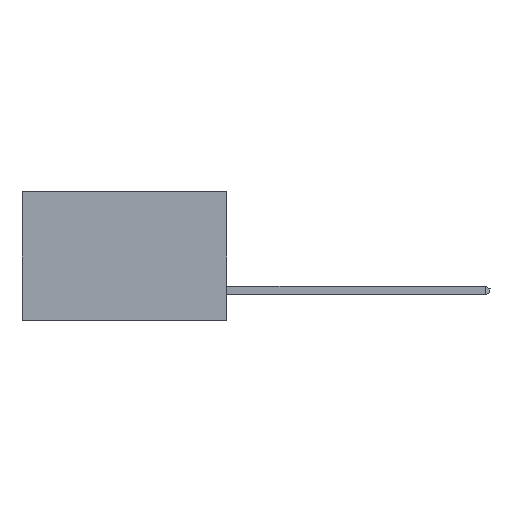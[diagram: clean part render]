
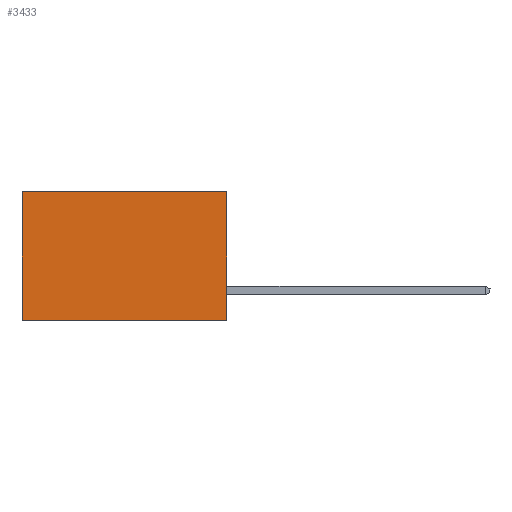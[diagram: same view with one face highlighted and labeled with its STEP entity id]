
A CAD part, left-side view. The second image highlights one B-rep face of the part: STEP entity #3433.
In plain terms, the highlighted planar face has unit normal (-1, 0, 0).
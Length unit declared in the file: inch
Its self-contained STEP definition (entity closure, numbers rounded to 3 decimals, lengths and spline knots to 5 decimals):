
#460 = ORIENTED_EDGE ( 'NONE', *, *, #3044, .F. ) ;
#635 = EDGE_CURVE ( 'NONE', #4662, #4402, #11869, .T. ) ;
#677 = ORIENTED_EDGE ( 'NONE', *, *, #10518, .T. ) ;
#2318 = AXIS2_PLACEMENT_3D ( 'NONE', #15394, #14809, #14238 ) ;
#2952 = VECTOR ( 'NONE', #11300, 39.37008 ) ;
#3044 = EDGE_CURVE ( 'NONE', #17168, #6443, #9224, .T. ) ;
#3433 = ADVANCED_FACE ( 'NONE', ( #16852 ), #17088, .F. ) ;
#4402 = VERTEX_POINT ( 'NONE', #13492 ) ;
#4662 = VERTEX_POINT ( 'NONE', #12354 ) ;
#5061 = VECTOR ( 'NONE', #13582, 39.37008 ) ;
#6443 = VERTEX_POINT ( 'NONE', #7314 ) ;
#7314 = CARTESIAN_POINT ( 'NONE',  ( 0.277, 0., -0.37 ) ) ;
#7480 = LINE ( 'NONE', #9941, #2952 ) ;
#7738 = EDGE_CURVE ( 'NONE', #6443, #4402, #7480, .T. ) ;
#7836 = VECTOR ( 'NONE', #7999, 39.37008 ) ;
#7954 = EDGE_LOOP ( 'NONE', ( #14583, #15411, #460, #677 ) ) ;
#7999 = DIRECTION ( 'NONE',  ( 0., 1., 0. ) ) ;
#9224 = LINE ( 'NONE', #13761, #5061 ) ;
#9941 = CARTESIAN_POINT ( 'NONE',  ( 0.277, 0., -0.37 ) ) ;
#10518 = EDGE_CURVE ( 'NONE', #17168, #4662, #11487, .T. ) ;
#11300 = DIRECTION ( 'NONE',  ( 0., 1., 0. ) ) ;
#11438 = VECTOR ( 'NONE', #17755, 39.37008 ) ;
#11487 = LINE ( 'NONE', #14865, #7836 ) ;
#11869 = LINE ( 'NONE', #16660, #11438 ) ;
#12354 = CARTESIAN_POINT ( 'NONE',  ( 0.277, 0.59, 0. ) ) ;
#13492 = CARTESIAN_POINT ( 'NONE',  ( 0.277, 0.59, -0.37 ) ) ;
#13582 = DIRECTION ( 'NONE',  ( 0., 0., -1. ) ) ;
#13761 = CARTESIAN_POINT ( 'NONE',  ( 0.277, 0., -0.37 ) ) ;
#14060 = CARTESIAN_POINT ( 'NONE',  ( 0.277, 0., 0. ) ) ;
#14238 = DIRECTION ( 'NONE',  ( 0., 0., -1. ) ) ;
#14583 = ORIENTED_EDGE ( 'NONE', *, *, #635, .T. ) ;
#14809 = DIRECTION ( 'NONE',  ( 1., 0., 0. ) ) ;
#14865 = CARTESIAN_POINT ( 'NONE',  ( 0.277, 0., 0. ) ) ;
#15394 = CARTESIAN_POINT ( 'NONE',  ( 0.277, 0., -0.37 ) ) ;
#15411 = ORIENTED_EDGE ( 'NONE', *, *, #7738, .F. ) ;
#16660 = CARTESIAN_POINT ( 'NONE',  ( 0.277, 0.59, -0.37 ) ) ;
#16852 = FACE_OUTER_BOUND ( 'NONE', #7954, .T. ) ;
#17088 = PLANE ( 'NONE',  #2318 ) ;
#17168 = VERTEX_POINT ( 'NONE', #14060 ) ;
#17755 = DIRECTION ( 'NONE',  ( 0., 0., -1. ) ) ;
